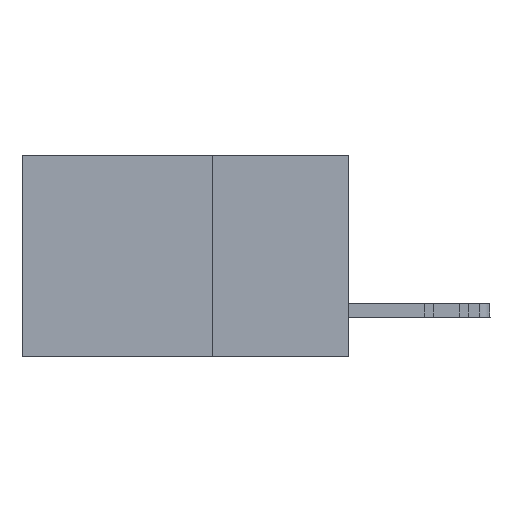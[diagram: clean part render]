
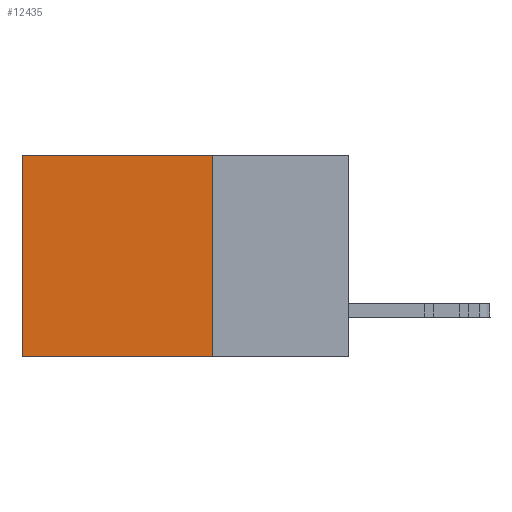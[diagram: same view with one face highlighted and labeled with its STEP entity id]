
A CAD part, left-side view. The second image highlights one B-rep face of the part: STEP entity #12435.
In plain terms, the highlighted planar face has unit normal (-1, 0, 0).
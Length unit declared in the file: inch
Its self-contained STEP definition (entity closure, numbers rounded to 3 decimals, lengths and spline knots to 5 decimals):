
#342 = VERTEX_POINT ( 'NONE', #17210 ) ;
#854 = VECTOR ( 'NONE', #8319, 39.37008 ) ;
#3835 = DIRECTION ( 'NONE',  ( 0., 0., -1. ) ) ;
#3863 = CARTESIAN_POINT ( 'NONE',  ( 0.298, 0.25, 0. ) ) ;
#4414 = ORIENTED_EDGE ( 'NONE', *, *, #4696, .T. ) ;
#4590 = ORIENTED_EDGE ( 'NONE', *, *, #9929, .F. ) ;
#4696 = EDGE_CURVE ( 'NONE', #27656, #26320, #17406, .T. ) ;
#6914 = EDGE_CURVE ( 'NONE', #26320, #342, #26119, .T. ) ;
#7678 = PLANE ( 'NONE',  #26083 ) ;
#7841 = CARTESIAN_POINT ( 'NONE',  ( 0.298, 0.6, 0. ) ) ;
#8319 = DIRECTION ( 'NONE',  ( 0., 1., 0. ) ) ;
#9403 = CARTESIAN_POINT ( 'NONE',  ( 0.298, 0.25, 0. ) ) ;
#9897 = EDGE_LOOP ( 'NONE', ( #17667, #18259, #4590, #4414 ) ) ;
#9929 = EDGE_CURVE ( 'NONE', #27656, #21286, #24869, .T. ) ;
#11693 = VECTOR ( 'NONE', #3835, 39.37008 ) ;
#12435 = ADVANCED_FACE ( 'NONE', ( #16497 ), #7678, .F. ) ;
#13140 = CARTESIAN_POINT ( 'NONE',  ( 0.298, 0.25, 0. ) ) ;
#14768 = LINE ( 'NONE', #23426, #17312 ) ;
#15189 = CARTESIAN_POINT ( 'NONE',  ( 0.298, 0.25, -0.37 ) ) ;
#15358 = CARTESIAN_POINT ( 'NONE',  ( 0.298, 0.6, 0. ) ) ;
#16115 = EDGE_CURVE ( 'NONE', #21286, #342, #14768, .T. ) ;
#16497 = FACE_OUTER_BOUND ( 'NONE', #9897, .T. ) ;
#17210 = CARTESIAN_POINT ( 'NONE',  ( 0.298, 0.6, -0.37 ) ) ;
#17312 = VECTOR ( 'NONE', #23970, 39.37008 ) ;
#17406 = LINE ( 'NONE', #26043, #854 ) ;
#17667 = ORIENTED_EDGE ( 'NONE', *, *, #6914, .T. ) ;
#18259 = ORIENTED_EDGE ( 'NONE', *, *, #16115, .F. ) ;
#20447 = VECTOR ( 'NONE', #24010, 39.37008 ) ;
#21286 = VERTEX_POINT ( 'NONE', #15189 ) ;
#22746 = DIRECTION ( 'NONE',  ( 0., 0., -1. ) ) ;
#23319 = DIRECTION ( 'NONE',  ( 1., 0., 0. ) ) ;
#23426 = CARTESIAN_POINT ( 'NONE',  ( 0.298, 0.25, -0.37 ) ) ;
#23970 = DIRECTION ( 'NONE',  ( 0., 1., 0. ) ) ;
#24010 = DIRECTION ( 'NONE',  ( 0., 0., -1. ) ) ;
#24869 = LINE ( 'NONE', #9403, #11693 ) ;
#26043 = CARTESIAN_POINT ( 'NONE',  ( 0.298, 0.25, 0. ) ) ;
#26083 = AXIS2_PLACEMENT_3D ( 'NONE', #3863, #23319, #22746 ) ;
#26119 = LINE ( 'NONE', #15358, #20447 ) ;
#26320 = VERTEX_POINT ( 'NONE', #7841 ) ;
#27656 = VERTEX_POINT ( 'NONE', #13140 ) ;
